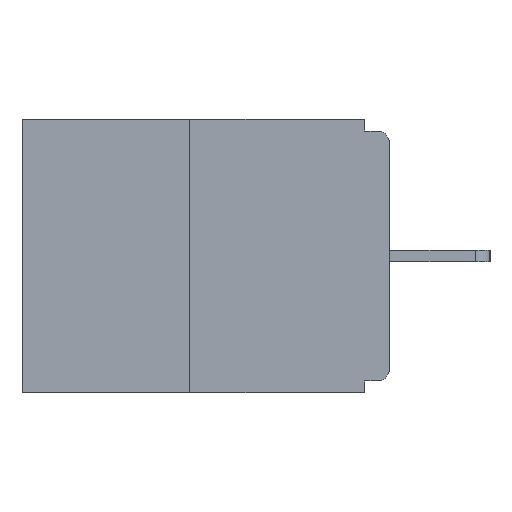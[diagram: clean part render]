
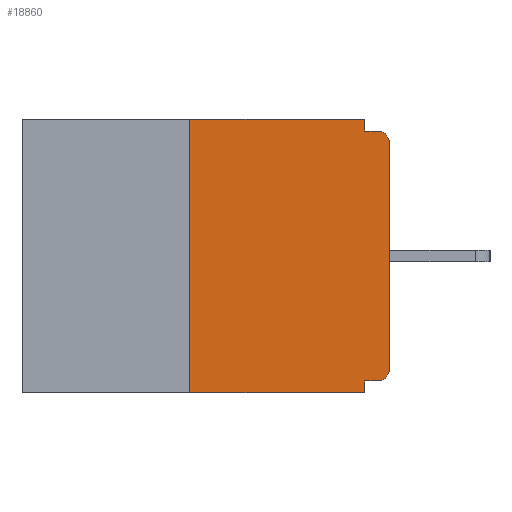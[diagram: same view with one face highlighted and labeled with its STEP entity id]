
A CAD part, left-side view. The second image highlights one B-rep face of the part: STEP entity #18860.
In plain terms, the highlighted planar face has unit normal (-1, 0, 0).
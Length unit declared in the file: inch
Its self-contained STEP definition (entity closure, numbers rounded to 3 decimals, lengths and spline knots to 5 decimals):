
#500 = DIRECTION ( 'NONE',  ( 0., -1., 0. ) ) ;
#558 = EDGE_CURVE ( 'NONE', #26952, #22351, #15217, .T. ) ;
#778 = VERTEX_POINT ( 'NONE', #22789 ) ;
#1048 = VECTOR ( 'NONE', #22172, 39.37008 ) ;
#1607 = VECTOR ( 'NONE', #21450, 39.37008 ) ;
#2084 = DIRECTION ( 'NONE',  ( 0., -1., 0. ) ) ;
#2629 = DIRECTION ( 'NONE',  ( 0., 0., -1. ) ) ;
#2630 = VERTEX_POINT ( 'NONE', #24264 ) ;
#2926 = AXIS2_PLACEMENT_3D ( 'NONE', #13768, #22209, #2629 ) ;
#3211 = DIRECTION ( 'NONE',  ( 1., 0., 0. ) ) ;
#3649 = DIRECTION ( 'NONE',  ( 0., 0., -1. ) ) ;
#4081 = VERTEX_POINT ( 'NONE', #22270 ) ;
#5415 = EDGE_CURVE ( 'NONE', #16191, #4081, #26471, .T. ) ;
#6094 = DIRECTION ( 'NONE',  ( 0., 0., -1. ) ) ;
#6242 = EDGE_CURVE ( 'NONE', #2630, #778, #13854, .T. ) ;
#6357 = ORIENTED_EDGE ( 'NONE', *, *, #6242, .T. ) ;
#7508 = ORIENTED_EDGE ( 'NONE', *, *, #17205, .T. ) ;
#7519 = VECTOR ( 'NONE', #2084, 39.37008 ) ;
#7930 = PLANE ( 'NONE',  #24833 ) ;
#8188 = DIRECTION ( 'NONE',  ( 0., 0., 1. ) ) ;
#8475 = VERTEX_POINT ( 'NONE', #23395 ) ;
#8527 = LINE ( 'NONE', #14951, #19272 ) ;
#8530 = EDGE_LOOP ( 'NONE', ( #16380, #22985, #18868, #10755, #26950, #6357, #15611, #7508, #14507, #26955 ) ) ;
#8533 = VECTOR ( 'NONE', #20929, 39.37008 ) ;
#8841 = VERTEX_POINT ( 'NONE', #23364 ) ;
#9904 = CARTESIAN_POINT ( 'NONE',  ( 0., 0.25, 0. ) ) ;
#9926 = CARTESIAN_POINT ( 'NONE',  ( 0., 0.46, 0. ) ) ;
#10194 = LINE ( 'NONE', #9904, #23084 ) ;
#10755 = ORIENTED_EDGE ( 'NONE', *, *, #16627, .F. ) ;
#10845 = CARTESIAN_POINT ( 'NONE',  ( 0., 0.031, -0.328 ) ) ;
#10980 = CARTESIAN_POINT ( 'NONE',  ( 0., 0.46, 0. ) ) ;
#12050 = CARTESIAN_POINT ( 'NONE',  ( 0., 0.031, -0.343 ) ) ;
#12205 = LINE ( 'NONE', #18920, #8533 ) ;
#12318 = EDGE_CURVE ( 'NONE', #2630, #14148, #17168, .T. ) ;
#12330 = DIRECTION ( 'NONE',  ( 0., 1., 0. ) ) ;
#13311 = DIRECTION ( 'NONE',  ( -1., 0., 0. ) ) ;
#13768 = CARTESIAN_POINT ( 'NONE',  ( 0., 0.015, -0.313 ) ) ;
#13811 = AXIS2_PLACEMENT_3D ( 'NONE', #15467, #13311, #22041 ) ;
#13854 = CIRCLE ( 'NONE', #2926, 0.015 ) ;
#14148 = VERTEX_POINT ( 'NONE', #10845 ) ;
#14507 = ORIENTED_EDGE ( 'NONE', *, *, #15303, .F. ) ;
#14578 = VECTOR ( 'NONE', #500, 39.37008 ) ;
#14951 = CARTESIAN_POINT ( 'NONE',  ( 0., 0.031, -0.343 ) ) ;
#15217 = LINE ( 'NONE', #17098, #7519 ) ;
#15303 = EDGE_CURVE ( 'NONE', #4081, #8475, #26676, .T. ) ;
#15467 = CARTESIAN_POINT ( 'NONE',  ( 0., 0.015, -0.03 ) ) ;
#15526 = CARTESIAN_POINT ( 'NONE',  ( 0., 0., -0.015 ) ) ;
#15611 = ORIENTED_EDGE ( 'NONE', *, *, #22378, .T. ) ;
#16191 = VERTEX_POINT ( 'NONE', #19005 ) ;
#16380 = ORIENTED_EDGE ( 'NONE', *, *, #21005, .F. ) ;
#16627 = EDGE_CURVE ( 'NONE', #14148, #22351, #8527, .T. ) ;
#17098 = CARTESIAN_POINT ( 'NONE',  ( 0., 0.46, -0.343 ) ) ;
#17168 = LINE ( 'NONE', #25890, #25478 ) ;
#17205 = EDGE_CURVE ( 'NONE', #21133, #8475, #25692, .T. ) ;
#18860 = ADVANCED_FACE ( 'NONE', ( #27500 ), #7930, .F. ) ;
#18868 = ORIENTED_EDGE ( 'NONE', *, *, #558, .T. ) ;
#18920 = CARTESIAN_POINT ( 'NONE',  ( 0., 0., 0. ) ) ;
#19005 = CARTESIAN_POINT ( 'NONE',  ( 0., 0.031, 0. ) ) ;
#19134 = CARTESIAN_POINT ( 'NONE',  ( 0., 0.25, -0.343 ) ) ;
#19272 = VECTOR ( 'NONE', #6094, 39.37008 ) ;
#19559 = LINE ( 'NONE', #10980, #1607 ) ;
#20929 = DIRECTION ( 'NONE',  ( 0., 0., 1. ) ) ;
#21005 = EDGE_CURVE ( 'NONE', #8841, #16191, #19559, .T. ) ;
#21133 = VERTEX_POINT ( 'NONE', #24383 ) ;
#21450 = DIRECTION ( 'NONE',  ( 0., -1., 0. ) ) ;
#21766 = EDGE_CURVE ( 'NONE', #26952, #8841, #10194, .T. ) ;
#22041 = DIRECTION ( 'NONE',  ( 0., 0., -1. ) ) ;
#22172 = DIRECTION ( 'NONE',  ( 0., 0., -1. ) ) ;
#22209 = DIRECTION ( 'NONE',  ( -1., 0., 0. ) ) ;
#22270 = CARTESIAN_POINT ( 'NONE',  ( 0., 0.031, -0.015 ) ) ;
#22351 = VERTEX_POINT ( 'NONE', #12050 ) ;
#22378 = EDGE_CURVE ( 'NONE', #778, #21133, #12205, .T. ) ;
#22595 = CARTESIAN_POINT ( 'NONE',  ( 0., 0.031, 0. ) ) ;
#22789 = CARTESIAN_POINT ( 'NONE',  ( 0., 0., -0.313 ) ) ;
#22985 = ORIENTED_EDGE ( 'NONE', *, *, #21766, .F. ) ;
#23084 = VECTOR ( 'NONE', #8188, 39.37008 ) ;
#23364 = CARTESIAN_POINT ( 'NONE',  ( 0., 0.25, 0. ) ) ;
#23395 = CARTESIAN_POINT ( 'NONE',  ( 0., 0.015, -0.015 ) ) ;
#24264 = CARTESIAN_POINT ( 'NONE',  ( 0., 0.015, -0.328 ) ) ;
#24383 = CARTESIAN_POINT ( 'NONE',  ( 0., 0., -0.03 ) ) ;
#24833 = AXIS2_PLACEMENT_3D ( 'NONE', #9926, #3211, #3649 ) ;
#25478 = VECTOR ( 'NONE', #12330, 39.37008 ) ;
#25692 = CIRCLE ( 'NONE', #13811, 0.015 ) ;
#25890 = CARTESIAN_POINT ( 'NONE',  ( 0., 0., -0.328 ) ) ;
#26471 = LINE ( 'NONE', #22595, #1048 ) ;
#26676 = LINE ( 'NONE', #15526, #14578 ) ;
#26950 = ORIENTED_EDGE ( 'NONE', *, *, #12318, .F. ) ;
#26952 = VERTEX_POINT ( 'NONE', #19134 ) ;
#26955 = ORIENTED_EDGE ( 'NONE', *, *, #5415, .F. ) ;
#27500 = FACE_OUTER_BOUND ( 'NONE', #8530, .T. ) ;
